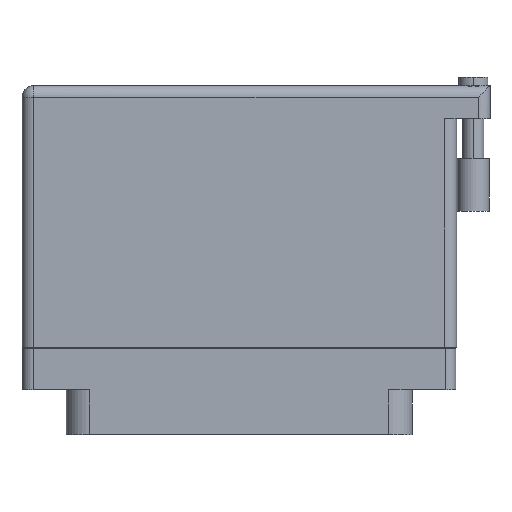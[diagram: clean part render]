
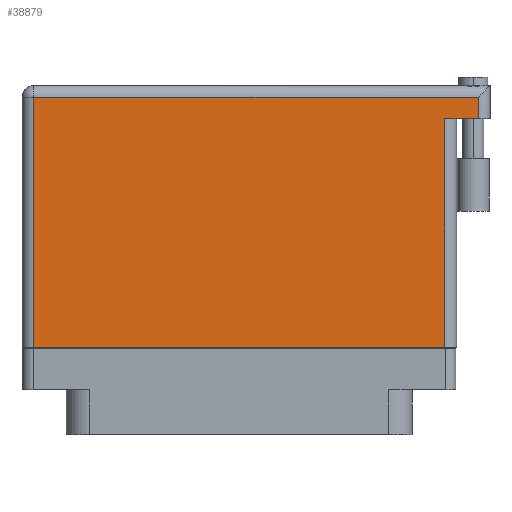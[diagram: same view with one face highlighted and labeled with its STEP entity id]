
A CAD part, front view. The second image highlights one B-rep face of the part: STEP entity #38879.
In plain terms, the highlighted face is planar.
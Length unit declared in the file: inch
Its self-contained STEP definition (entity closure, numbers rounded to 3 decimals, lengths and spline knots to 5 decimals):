
#245 = CARTESIAN_POINT ( 'NONE',  ( 1.23, 1.269, 0.4495 ) ) ;
#1460 = EDGE_CURVE ( 'NONE', #4316, #19688, #15592, .T. ) ;
#1839 = EDGE_CURVE ( 'NONE', #30427, #4316, #46845, .T. ) ;
#2818 = DIRECTION ( 'NONE',  ( -1., 0., 0. ) ) ;
#3450 = CARTESIAN_POINT ( 'NONE',  ( -1.23, -0.1, 0.4495 ) ) ;
#4185 = LINE ( 'NONE', #245, #7537 ) ;
#4316 = VERTEX_POINT ( 'NONE', #4416 ) ;
#4416 = CARTESIAN_POINT ( 'NONE',  ( 1.43, 1.396, 0.4495 ) ) ;
#4919 = VERTEX_POINT ( 'NONE', #10559 ) ;
#7537 = VECTOR ( 'NONE', #27696, 39.37008 ) ;
#8558 = ORIENTED_EDGE ( 'NONE', *, *, #42268, .T. ) ;
#10559 = CARTESIAN_POINT ( 'NONE',  ( -1.23, -0.1, 0.4495 ) ) ;
#10901 = ORIENTED_EDGE ( 'NONE', *, *, #1460, .T. ) ;
#11074 = DIRECTION ( 'NONE',  ( 0., 1., 0. ) ) ;
#11368 = VECTOR ( 'NONE', #34540, 39.37008 ) ;
#11709 = LINE ( 'NONE', #12199, #40044 ) ;
#12161 = CARTESIAN_POINT ( 'NONE',  ( -1.3, 1.396, 0.4495 ) ) ;
#12199 = CARTESIAN_POINT ( 'NONE',  ( -1.3, -0.1, 0.4495 ) ) ;
#14593 = EDGE_CURVE ( 'NONE', #19688, #4919, #31683, .T. ) ;
#14643 = DIRECTION ( 'NONE',  ( 1., 0., 0. ) ) ;
#15592 = LINE ( 'NONE', #12161, #42113 ) ;
#18033 = EDGE_LOOP ( 'NONE', ( #36465, #8558, #20147, #49950, #10901, #34115 ) ) ;
#19688 = VERTEX_POINT ( 'NONE', #25640 ) ;
#20147 = ORIENTED_EDGE ( 'NONE', *, *, #39006, .F. ) ;
#20442 = VECTOR ( 'NONE', #11074, 39.37008 ) ;
#23564 = DIRECTION ( 'NONE',  ( -1., 0., 0. ) ) ;
#25640 = CARTESIAN_POINT ( 'NONE',  ( -1.23, 1.396, 0.4495 ) ) ;
#25739 = VECTOR ( 'NONE', #2818, 39.37008 ) ;
#27605 = DIRECTION ( 'NONE',  ( -1., 0., 0. ) ) ;
#27696 = DIRECTION ( 'NONE',  ( 0., 1., 0. ) ) ;
#30031 = LINE ( 'NONE', #30545, #25739 ) ;
#30427 = VERTEX_POINT ( 'NONE', #47810 ) ;
#30545 = CARTESIAN_POINT ( 'NONE',  ( 1.5, 1.269, 0.4495 ) ) ;
#31683 = LINE ( 'NONE', #3450, #11368 ) ;
#31729 = CARTESIAN_POINT ( 'NONE',  ( 1.43, 1.466, 0.4495 ) ) ;
#34085 = VERTEX_POINT ( 'NONE', #39877 ) ;
#34115 = ORIENTED_EDGE ( 'NONE', *, *, #14593, .T. ) ;
#34540 = DIRECTION ( 'NONE',  ( 0., -1., 0. ) ) ;
#34836 = FACE_OUTER_BOUND ( 'NONE', #18033, .T. ) ;
#35602 = CARTESIAN_POINT ( 'NONE',  ( -1.3, 1.466, 0.4495 ) ) ;
#35974 = VERTEX_POINT ( 'NONE', #47623 ) ;
#36465 = ORIENTED_EDGE ( 'NONE', *, *, #41735, .T. ) ;
#38280 = AXIS2_PLACEMENT_3D ( 'NONE', #35602, #42891, #23564 ) ;
#38879 = ADVANCED_FACE ( 'NONE', ( #34836 ), #47051, .F. ) ;
#39006 = EDGE_CURVE ( 'NONE', #30427, #35974, #30031, .T. ) ;
#39877 = CARTESIAN_POINT ( 'NONE',  ( 1.23, -0.1, 0.4495 ) ) ;
#40044 = VECTOR ( 'NONE', #14643, 39.37008 ) ;
#41735 = EDGE_CURVE ( 'NONE', #4919, #34085, #11709, .T. ) ;
#42113 = VECTOR ( 'NONE', #27605, 39.37008 ) ;
#42268 = EDGE_CURVE ( 'NONE', #34085, #35974, #4185, .T. ) ;
#42891 = DIRECTION ( 'NONE',  ( 0., 0., -1. ) ) ;
#46845 = LINE ( 'NONE', #31729, #20442 ) ;
#47051 = PLANE ( 'NONE',  #38280 ) ;
#47623 = CARTESIAN_POINT ( 'NONE',  ( 1.23, 1.269, 0.4495 ) ) ;
#47810 = CARTESIAN_POINT ( 'NONE',  ( 1.43, 1.269, 0.4495 ) ) ;
#49950 = ORIENTED_EDGE ( 'NONE', *, *, #1839, .T. ) ;
